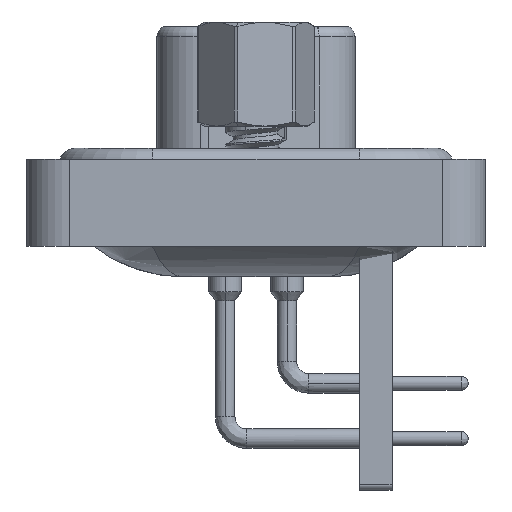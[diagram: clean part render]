
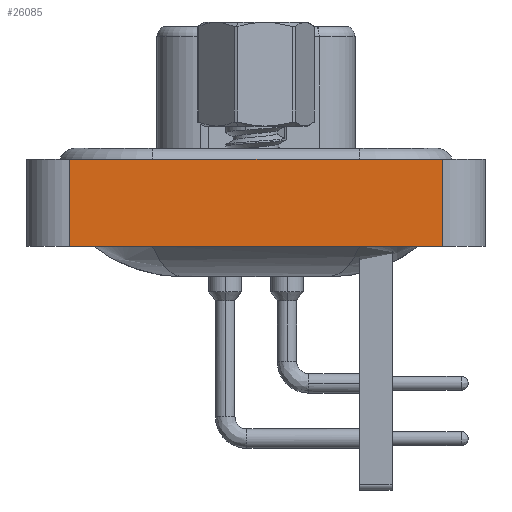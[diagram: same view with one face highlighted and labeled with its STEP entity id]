
A CAD part, left-side view. The second image highlights one B-rep face of the part: STEP entity #26085.
In plain terms, the highlighted planar face has unit normal (-1, 0, 0).
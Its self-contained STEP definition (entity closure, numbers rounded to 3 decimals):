
#826 = VERTEX_POINT ( 'NONE', #17230 ) ;
#832 = LINE ( 'NONE', #24417, #9632 ) ;
#1768 = CARTESIAN_POINT ( 'NONE',  ( -7.35, -8.55, 0.4 ) ) ;
#2134 = CARTESIAN_POINT ( 'NONE',  ( -7.35, -8.55, -3.6 ) ) ;
#2299 = LINE ( 'NONE', #23155, #20340 ) ;
#3199 = EDGE_LOOP ( 'NONE', ( #26329, #13169, #18385, #4257 ) ) ;
#4257 = ORIENTED_EDGE ( 'NONE', *, *, #13687, .T. ) ;
#5982 = EDGE_CURVE ( 'NONE', #8455, #18447, #2299, .T. ) ;
#6715 = CARTESIAN_POINT ( 'NONE',  ( -7.35, -8.55, -3.6 ) ) ;
#7136 = CARTESIAN_POINT ( 'NONE',  ( -7.35, -8.55, -3.6 ) ) ;
#7756 = DIRECTION ( 'NONE',  ( 0., 0., 1. ) ) ;
#8059 = EDGE_CURVE ( 'NONE', #25667, #18447, #29930, .T. ) ;
#8455 = VERTEX_POINT ( 'NONE', #31793 ) ;
#8551 = EDGE_CURVE ( 'NONE', #826, #8455, #832, .T. ) ;
#9632 = VECTOR ( 'NONE', #14337, 1000. ) ;
#12267 = VECTOR ( 'NONE', #24978, 1000. ) ;
#12544 = DIRECTION ( 'NONE',  ( -1., 0., 0. ) ) ;
#12718 = DIRECTION ( 'NONE',  ( 0., -1., 0. ) ) ;
#12882 = PLANE ( 'NONE',  #23533 ) ;
#13169 = ORIENTED_EDGE ( 'NONE', *, *, #5982, .F. ) ;
#13687 = EDGE_CURVE ( 'NONE', #826, #25667, #17581, .T. ) ;
#14337 = DIRECTION ( 'NONE',  ( 0., 0., 1. ) ) ;
#14538 = CARTESIAN_POINT ( 'NONE',  ( -7.35, -8.55, -3.6 ) ) ;
#15006 = DIRECTION ( 'NONE',  ( 0., -1., 0. ) ) ;
#17230 = CARTESIAN_POINT ( 'NONE',  ( -7.35, 8.55, -3.6 ) ) ;
#17581 = LINE ( 'NONE', #7136, #33152 ) ;
#18385 = ORIENTED_EDGE ( 'NONE', *, *, #8551, .F. ) ;
#18447 = VERTEX_POINT ( 'NONE', #1768 ) ;
#20340 = VECTOR ( 'NONE', #12718, 1000. ) ;
#20936 = FACE_OUTER_BOUND ( 'NONE', #3199, .T. ) ;
#23155 = CARTESIAN_POINT ( 'NONE',  ( -7.35, -8.55, 0.4 ) ) ;
#23533 = AXIS2_PLACEMENT_3D ( 'NONE', #2134, #12544, #7756 ) ;
#24417 = CARTESIAN_POINT ( 'NONE',  ( -7.35, 8.55, -3.6 ) ) ;
#24978 = DIRECTION ( 'NONE',  ( 0., 0., 1. ) ) ;
#25667 = VERTEX_POINT ( 'NONE', #6715 ) ;
#26085 = ADVANCED_FACE ( 'NONE', ( #20936 ), #12882, .T. ) ;
#26329 = ORIENTED_EDGE ( 'NONE', *, *, #8059, .T. ) ;
#29930 = LINE ( 'NONE', #14538, #12267 ) ;
#31793 = CARTESIAN_POINT ( 'NONE',  ( -7.35, 8.55, 0.4 ) ) ;
#33152 = VECTOR ( 'NONE', #15006, 1000. ) ;
